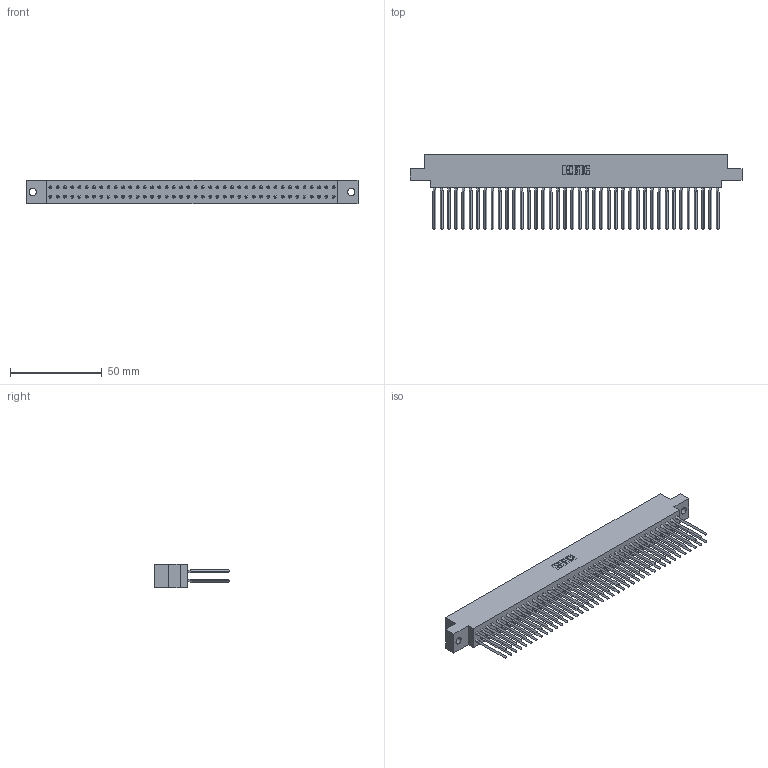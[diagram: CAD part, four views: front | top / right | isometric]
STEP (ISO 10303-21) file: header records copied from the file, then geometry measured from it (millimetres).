
FILE_DESCRIPTION (( 'STEP AP203' ), '1' );
FILE_NAME ('317-080-543-804.STEP', '2020-02-28T09:25:31', ( '' ), ( '' ), 'SwSTEP 2.0', 'SolidWorks 2016', '' );
FILE_SCHEMA (( 'CONFIG_CONTROL_DESIGN' ));
Length unit declared in the file: inch
Products named in the file (3): 317-290-001_543; 317 Part_.156 Dia - TH; 317-080-543-804
Assembly tree (81 placements, depth 2):
  317-080-543-804
    317 Part_.156 Dia - TH
    317-290-001_543  x80
Bounding box: 181.2 x 41.15 x 12.7 mm (x, y, z)
Volume: 30654.3 mm3; surface area: 46252.2 mm2
Topology: 81 solids, 81 shells, 7222 faces, 20035 edges, 12902 vertices
Faces by surface type: plane 5898, cylinder 1004, bspline 320
Entity records: 58102 total; most frequent: CARTESIAN_POINT 10551, ORIENTED_EDGE 10050, DIRECTION 8383, EDGE_CURVE 5025, LINE 4769, VECTOR 4769, VERTEX_POINT 3343, AXIS2_PLACEMENT_3D 1807
